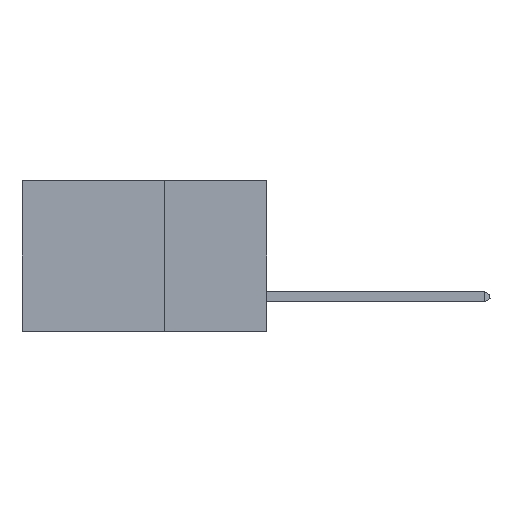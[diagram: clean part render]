
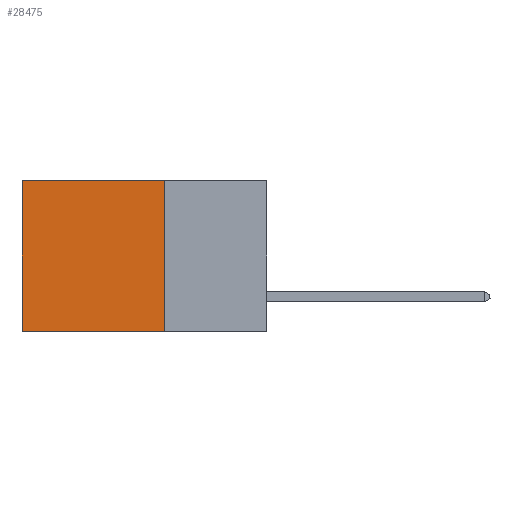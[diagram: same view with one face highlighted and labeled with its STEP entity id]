
A CAD part, left-side view. The second image highlights one B-rep face of the part: STEP entity #28475.
In plain terms, the highlighted planar face has unit normal (-1, 0, 0).
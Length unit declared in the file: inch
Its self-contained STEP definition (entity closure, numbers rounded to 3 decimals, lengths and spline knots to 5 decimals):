
#670 = EDGE_CURVE ( 'NONE', #6608, #8805, #37611, .T. ) ;
#3320 = EDGE_CURVE ( 'NONE', #40248, #8805, #34758, .T. ) ;
#4897 = CARTESIAN_POINT ( 'NONE',  ( 0.2875, 0.25, 0. ) ) ;
#5527 = ORIENTED_EDGE ( 'NONE', *, *, #3320, .F. ) ;
#5650 = CARTESIAN_POINT ( 'NONE',  ( 0.2875, 0.25, -0.37 ) ) ;
#6608 = VERTEX_POINT ( 'NONE', #33422 ) ;
#7490 = EDGE_CURVE ( 'NONE', #28574, #6608, #15812, .T. ) ;
#7929 = PLANE ( 'NONE',  #35320 ) ;
#8484 = ORIENTED_EDGE ( 'NONE', *, *, #670, .T. ) ;
#8592 = DIRECTION ( 'NONE',  ( 0., 1., 0. ) ) ;
#8805 = VERTEX_POINT ( 'NONE', #11623 ) ;
#9102 = VECTOR ( 'NONE', #35982, 39.37008 ) ;
#9405 = ORIENTED_EDGE ( 'NONE', *, *, #7490, .T. ) ;
#10199 = LINE ( 'NONE', #42840, #9102 ) ;
#11623 = CARTESIAN_POINT ( 'NONE',  ( 0.2875, 0.6, -0.37 ) ) ;
#12439 = FACE_OUTER_BOUND ( 'NONE', #40599, .T. ) ;
#13072 = VECTOR ( 'NONE', #33752, 39.37008 ) ;
#15812 = LINE ( 'NONE', #38025, #37666 ) ;
#16739 = VECTOR ( 'NONE', #8592, 39.37008 ) ;
#18721 = DIRECTION ( 'NONE',  ( 0., 0., -1. ) ) ;
#24262 = ORIENTED_EDGE ( 'NONE', *, *, #35555, .F. ) ;
#26097 = CARTESIAN_POINT ( 'NONE',  ( 0.2875, 0.25, -0.37 ) ) ;
#28475 = ADVANCED_FACE ( 'NONE', ( #12439 ), #7929, .F. ) ;
#28574 = VERTEX_POINT ( 'NONE', #36249 ) ;
#33422 = CARTESIAN_POINT ( 'NONE',  ( 0.2875, 0.6, 0. ) ) ;
#33458 = CARTESIAN_POINT ( 'NONE',  ( 0.2875, 0.6, 0. ) ) ;
#33752 = DIRECTION ( 'NONE',  ( 0., 0., -1. ) ) ;
#34758 = LINE ( 'NONE', #26097, #16739 ) ;
#35320 = AXIS2_PLACEMENT_3D ( 'NONE', #4897, #39032, #18721 ) ;
#35555 = EDGE_CURVE ( 'NONE', #28574, #40248, #10199, .T. ) ;
#35982 = DIRECTION ( 'NONE',  ( 0., 0., -1. ) ) ;
#36249 = CARTESIAN_POINT ( 'NONE',  ( 0.2875, 0.25, 0. ) ) ;
#37611 = LINE ( 'NONE', #33458, #13072 ) ;
#37666 = VECTOR ( 'NONE', #45059, 39.37008 ) ;
#38025 = CARTESIAN_POINT ( 'NONE',  ( 0.2875, 0.25, 0. ) ) ;
#39032 = DIRECTION ( 'NONE',  ( 1., 0., 0. ) ) ;
#40248 = VERTEX_POINT ( 'NONE', #5650 ) ;
#40599 = EDGE_LOOP ( 'NONE', ( #8484, #5527, #24262, #9405 ) ) ;
#42840 = CARTESIAN_POINT ( 'NONE',  ( 0.2875, 0.25, 0. ) ) ;
#45059 = DIRECTION ( 'NONE',  ( 0., 1., 0. ) ) ;
